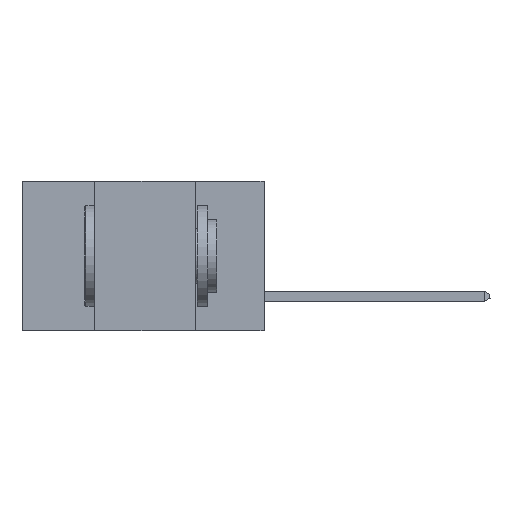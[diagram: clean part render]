
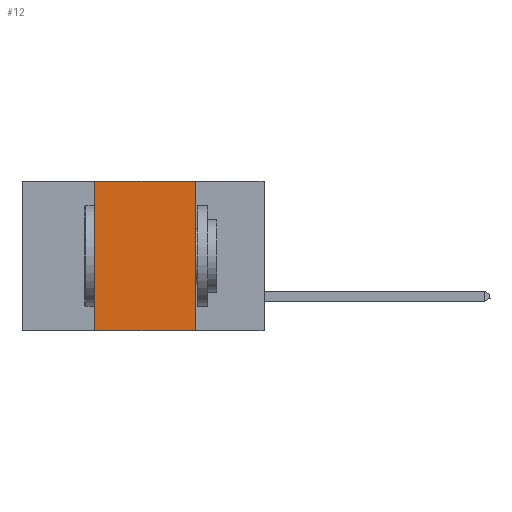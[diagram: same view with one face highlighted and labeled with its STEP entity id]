
A CAD part, left-side view. The second image highlights one B-rep face of the part: STEP entity #12.
In plain terms, the highlighted planar face has unit normal (-1, 0, 0).
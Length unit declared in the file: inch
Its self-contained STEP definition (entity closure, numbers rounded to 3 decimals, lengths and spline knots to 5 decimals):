
#12 = ADVANCED_FACE ( 'NONE', ( #9231 ), #7760, .F. ) ;
#23 = ORIENTED_EDGE ( 'NONE', *, *, #6576, .T. ) ;
#147 = VERTEX_POINT ( 'NONE', #4916 ) ;
#1012 = DIRECTION ( 'NONE',  ( 0., -1., 0. ) ) ;
#1858 = CARTESIAN_POINT ( 'NONE',  ( 0., 0.6, 0. ) ) ;
#2125 = CARTESIAN_POINT ( 'NONE',  ( 0., 0.6, -0.37 ) ) ;
#2172 = VECTOR ( 'NONE', #8010, 39.37008 ) ;
#2353 = VECTOR ( 'NONE', #10880, 39.37008 ) ;
#2607 = CARTESIAN_POINT ( 'NONE',  ( 0., 0.17, 0. ) ) ;
#3010 = VERTEX_POINT ( 'NONE', #8445 ) ;
#3413 = CARTESIAN_POINT ( 'NONE',  ( 0., 0.17, -0.37 ) ) ;
#3613 = AXIS2_PLACEMENT_3D ( 'NONE', #11754, #4728, #9796 ) ;
#3702 = LINE ( 'NONE', #9149, #2172 ) ;
#3714 = ORIENTED_EDGE ( 'NONE', *, *, #8206, .F. ) ;
#4121 = VERTEX_POINT ( 'NONE', #6696 ) ;
#4581 = DIRECTION ( 'NONE',  ( 0., 0., -1. ) ) ;
#4722 = VECTOR ( 'NONE', #4581, 39.37008 ) ;
#4728 = DIRECTION ( 'NONE',  ( 1., 0., 0. ) ) ;
#4916 = CARTESIAN_POINT ( 'NONE',  ( 0., 0.42, 0. ) ) ;
#6154 = LINE ( 'NONE', #2607, #4722 ) ;
#6448 = EDGE_CURVE ( 'NONE', #147, #3010, #8479, .T. ) ;
#6576 = EDGE_CURVE ( 'NONE', #4121, #9701, #8174, .T. ) ;
#6696 = CARTESIAN_POINT ( 'NONE',  ( 0., 0.42, -0.37 ) ) ;
#7760 = PLANE ( 'NONE',  #3613 ) ;
#8010 = DIRECTION ( 'NONE',  ( 0., 0., 1. ) ) ;
#8096 = ORIENTED_EDGE ( 'NONE', *, *, #6448, .F. ) ;
#8174 = LINE ( 'NONE', #2125, #8337 ) ;
#8206 = EDGE_CURVE ( 'NONE', #4121, #147, #3702, .T. ) ;
#8337 = VECTOR ( 'NONE', #1012, 39.37008 ) ;
#8445 = CARTESIAN_POINT ( 'NONE',  ( 0., 0.17, 0. ) ) ;
#8479 = LINE ( 'NONE', #1858, #2353 ) ;
#8774 = ORIENTED_EDGE ( 'NONE', *, *, #11229, .F. ) ;
#9149 = CARTESIAN_POINT ( 'NONE',  ( 0., 0.42, 0. ) ) ;
#9231 = FACE_OUTER_BOUND ( 'NONE', #11481, .T. ) ;
#9701 = VERTEX_POINT ( 'NONE', #3413 ) ;
#9796 = DIRECTION ( 'NONE',  ( 0., 0., -1. ) ) ;
#10880 = DIRECTION ( 'NONE',  ( 0., -1., 0. ) ) ;
#11229 = EDGE_CURVE ( 'NONE', #3010, #9701, #6154, .T. ) ;
#11481 = EDGE_LOOP ( 'NONE', ( #8774, #8096, #3714, #23 ) ) ;
#11754 = CARTESIAN_POINT ( 'NONE',  ( 0., 0.6, 0. ) ) ;
